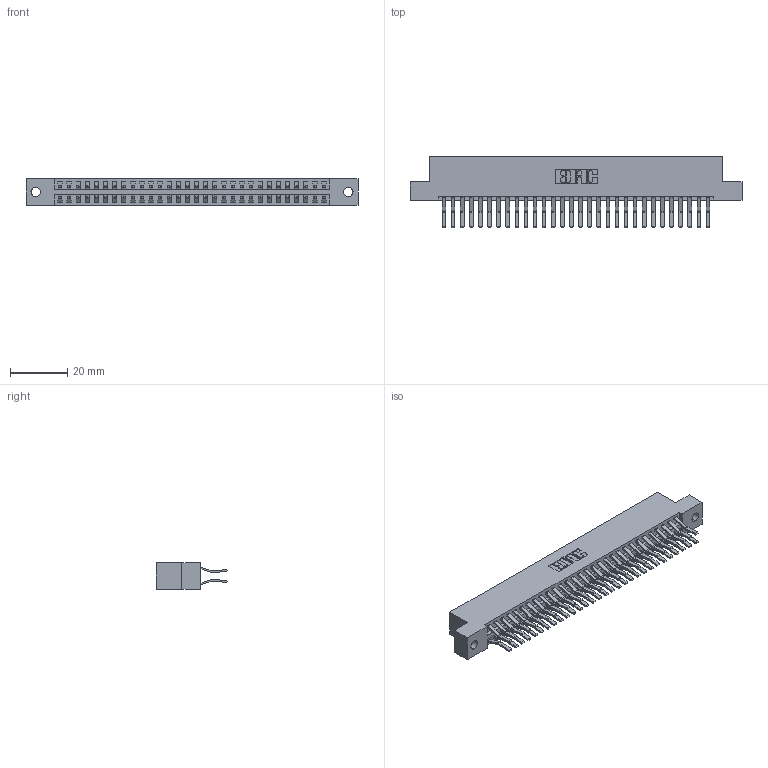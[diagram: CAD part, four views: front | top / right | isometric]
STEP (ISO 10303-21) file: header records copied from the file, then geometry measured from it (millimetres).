
FILE_DESCRIPTION (( 'STEP AP203' ), '1' );
FILE_NAME ('396-060-560-202.STEP', '2019-10-30T16:53:16', ( '' ), ( '' ), 'SwSTEP 2.0', 'SolidWorks 2016', '' );
FILE_SCHEMA (( 'CONFIG_CONTROL_DESIGN' ));
Length unit declared in the file: inch
Products named in the file (3): 396-060-560-202; 346 Part_Flush Mounting Lugs - 0.128 Dia; 345-292-001_560 Tail
Assembly tree (61 placements, depth 2):
  396-060-560-202
    346 Part_Flush Mounting Lugs - 0.128 Dia
    345-292-001_560 Tail  x60
Bounding box: 115.82 x 24.78 x 9.4 mm (x, y, z)
Volume: 11557.7 mm3; surface area: 16478.2 mm2
Topology: 61 solids, 61 shells, 3362 faces, 9989 edges, 6578 vertices
Faces by surface type: plane 2176, cylinder 1186
Entity records: 21285 total; most frequent: CARTESIAN_POINT 3524, ORIENTED_EDGE 3458, DIRECTION 3161, EDGE_CURVE 1729, VECTOR 1473, LINE 1473, VERTEX_POINT 1150, AXIS2_PLACEMENT_3D 844
